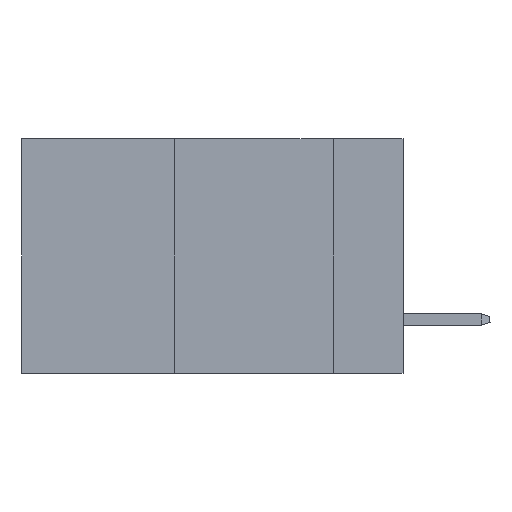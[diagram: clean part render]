
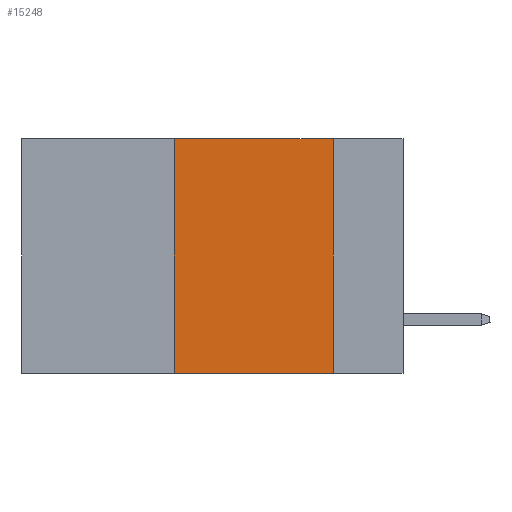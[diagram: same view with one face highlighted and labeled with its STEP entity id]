
A CAD part, left-side view. The second image highlights one B-rep face of the part: STEP entity #15248.
In plain terms, the highlighted planar face has unit normal (-1, 0, 0).
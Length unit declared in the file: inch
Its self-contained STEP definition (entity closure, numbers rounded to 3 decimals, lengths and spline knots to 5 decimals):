
#149 = DIRECTION ( 'NONE',  ( 0., 0., 1. ) ) ;
#217 = DIRECTION ( 'NONE',  ( 0., 0., -1. ) ) ;
#300 = VECTOR ( 'NONE', #217, 39.37008 ) ;
#728 = FACE_OUTER_BOUND ( 'NONE', #5876, .T. ) ;
#2715 = ORIENTED_EDGE ( 'NONE', *, *, #10309, .F. ) ;
#4103 = CARTESIAN_POINT ( 'NONE',  ( 0., 0.36, 0. ) ) ;
#5246 = CARTESIAN_POINT ( 'NONE',  ( 0., 0.11, -0.37 ) ) ;
#5876 = EDGE_LOOP ( 'NONE', ( #2715, #35821, #23428, #25828 ) ) ;
#7798 = PLANE ( 'NONE',  #40349 ) ;
#9810 = LINE ( 'NONE', #12656, #20275 ) ;
#10309 = EDGE_CURVE ( 'NONE', #10354, #35511, #26646, .T. ) ;
#10354 = VERTEX_POINT ( 'NONE', #42425 ) ;
#12656 = CARTESIAN_POINT ( 'NONE',  ( 0., 0.6, 0. ) ) ;
#14402 = EDGE_CURVE ( 'NONE', #42584, #35511, #16476, .T. ) ;
#15248 = ADVANCED_FACE ( 'NONE', ( #728 ), #7798, .F. ) ;
#16192 = CARTESIAN_POINT ( 'NONE',  ( 0., 0.36, 0. ) ) ;
#16476 = LINE ( 'NONE', #42911, #27615 ) ;
#20275 = VECTOR ( 'NONE', #40395, 39.37008 ) ;
#23428 = ORIENTED_EDGE ( 'NONE', *, *, #42041, .F. ) ;
#25828 = ORIENTED_EDGE ( 'NONE', *, *, #14402, .T. ) ;
#26646 = LINE ( 'NONE', #33705, #300 ) ;
#27615 = VECTOR ( 'NONE', #33471, 39.37008 ) ;
#27614 = CARTESIAN_POINT ( 'NONE',  ( 0., 0.6, 0. ) ) ;
#33471 = DIRECTION ( 'NONE',  ( 0., -1., 0. ) ) ;
#33705 = CARTESIAN_POINT ( 'NONE',  ( 0., 0.11, 0. ) ) ;
#34554 = VERTEX_POINT ( 'NONE', #16192 ) ;
#34873 = DIRECTION ( 'NONE',  ( 0., 0., -1. ) ) ;
#35511 = VERTEX_POINT ( 'NONE', #5246 ) ;
#35726 = VECTOR ( 'NONE', #149, 39.37008 ) ;
#35821 = ORIENTED_EDGE ( 'NONE', *, *, #43436, .F. ) ;
#36934 = LINE ( 'NONE', #4103, #35726 ) ;
#39191 = CARTESIAN_POINT ( 'NONE',  ( 0., 0.36, -0.37 ) ) ;
#40349 = AXIS2_PLACEMENT_3D ( 'NONE', #27614, #41023, #34873 ) ;
#40395 = DIRECTION ( 'NONE',  ( 0., -1., 0. ) ) ;
#41023 = DIRECTION ( 'NONE',  ( 1., 0., 0. ) ) ;
#42041 = EDGE_CURVE ( 'NONE', #42584, #34554, #36934, .T. ) ;
#42425 = CARTESIAN_POINT ( 'NONE',  ( 0., 0.11, 0. ) ) ;
#42584 = VERTEX_POINT ( 'NONE', #39191 ) ;
#42911 = CARTESIAN_POINT ( 'NONE',  ( 0., 0.6, -0.37 ) ) ;
#43436 = EDGE_CURVE ( 'NONE', #34554, #10354, #9810, .T. ) ;
